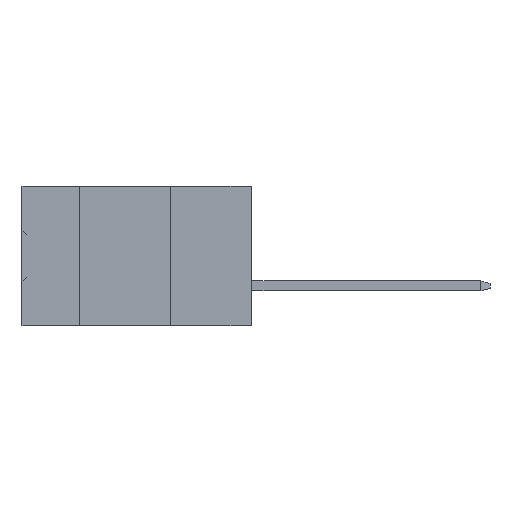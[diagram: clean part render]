
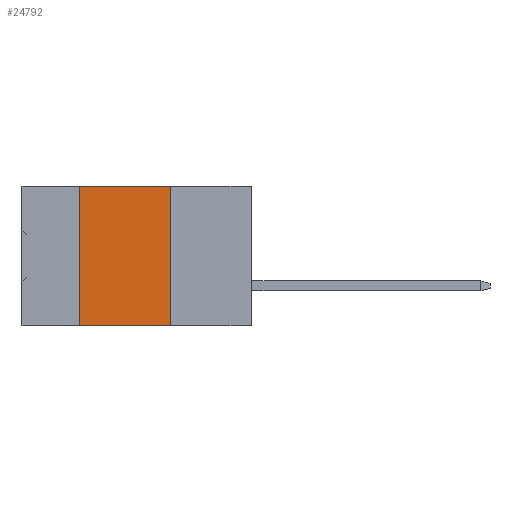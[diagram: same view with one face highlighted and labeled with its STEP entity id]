
A CAD part, left-side view. The second image highlights one B-rep face of the part: STEP entity #24792.
In plain terms, the highlighted planar face has unit normal (-1, 0, 0).
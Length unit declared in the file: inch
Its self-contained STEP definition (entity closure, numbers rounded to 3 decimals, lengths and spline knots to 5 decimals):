
#3236 = VERTEX_POINT ( 'NONE', #30684 ) ;
#4495 = LINE ( 'NONE', #17122, #16026 ) ;
#4733 = VECTOR ( 'NONE', #20106, 39.37008 ) ;
#5784 = DIRECTION ( 'NONE',  ( 1., 0., 0. ) ) ;
#6304 = VERTEX_POINT ( 'NONE', #18278 ) ;
#6764 = ORIENTED_EDGE ( 'NONE', *, *, #15198, .F. ) ;
#7258 = CARTESIAN_POINT ( 'NONE',  ( 0., 0.54, -0.437 ) ) ;
#7916 = EDGE_LOOP ( 'NONE', ( #25712, #12451, #6764, #14941 ) ) ;
#8547 = VERTEX_POINT ( 'NONE', #17855 ) ;
#9058 = CARTESIAN_POINT ( 'NONE',  ( 0., 0.254, -0.437 ) ) ;
#9078 = VECTOR ( 'NONE', #16532, 39.37008 ) ;
#9585 = DIRECTION ( 'NONE',  ( 0., -1., 0. ) ) ;
#10941 = AXIS2_PLACEMENT_3D ( 'NONE', #31538, #5784, #23552 ) ;
#12451 = ORIENTED_EDGE ( 'NONE', *, *, #30504, .F. ) ;
#13415 = PLANE ( 'NONE',  #10941 ) ;
#14053 = CARTESIAN_POINT ( 'NONE',  ( 0., 0.72, 0. ) ) ;
#14218 = EDGE_CURVE ( 'NONE', #3236, #8547, #14704, .T. ) ;
#14704 = LINE ( 'NONE', #9058, #9078 ) ;
#14941 = ORIENTED_EDGE ( 'NONE', *, *, #32725, .T. ) ;
#15198 = EDGE_CURVE ( 'NONE', #30686, #6304, #4495, .T. ) ;
#16026 = VECTOR ( 'NONE', #32602, 39.37008 ) ;
#16532 = DIRECTION ( 'NONE',  ( 0., 0., -1. ) ) ;
#17122 = CARTESIAN_POINT ( 'NONE',  ( 0., 0.54, -0.437 ) ) ;
#17855 = CARTESIAN_POINT ( 'NONE',  ( 0., 0.254, -0.437 ) ) ;
#18278 = CARTESIAN_POINT ( 'NONE',  ( 0., 0.54, 0. ) ) ;
#19618 = LINE ( 'NONE', #29807, #4733 ) ;
#20106 = DIRECTION ( 'NONE',  ( 0., -1., 0. ) ) ;
#21874 = LINE ( 'NONE', #14053, #24485 ) ;
#23552 = DIRECTION ( 'NONE',  ( 0., 0., -1. ) ) ;
#24485 = VECTOR ( 'NONE', #9585, 39.37008 ) ;
#24792 = ADVANCED_FACE ( 'NONE', ( #28729 ), #13415, .F. ) ;
#25712 = ORIENTED_EDGE ( 'NONE', *, *, #14218, .F. ) ;
#28729 = FACE_OUTER_BOUND ( 'NONE', #7916, .T. ) ;
#29807 = CARTESIAN_POINT ( 'NONE',  ( 0., 0.72, -0.437 ) ) ;
#30504 = EDGE_CURVE ( 'NONE', #6304, #3236, #21874, .T. ) ;
#30684 = CARTESIAN_POINT ( 'NONE',  ( 0., 0.254, 0. ) ) ;
#30686 = VERTEX_POINT ( 'NONE', #7258 ) ;
#31538 = CARTESIAN_POINT ( 'NONE',  ( 0., 0.72, 0. ) ) ;
#32602 = DIRECTION ( 'NONE',  ( 0., 0., 1. ) ) ;
#32725 = EDGE_CURVE ( 'NONE', #30686, #8547, #19618, .T. ) ;
